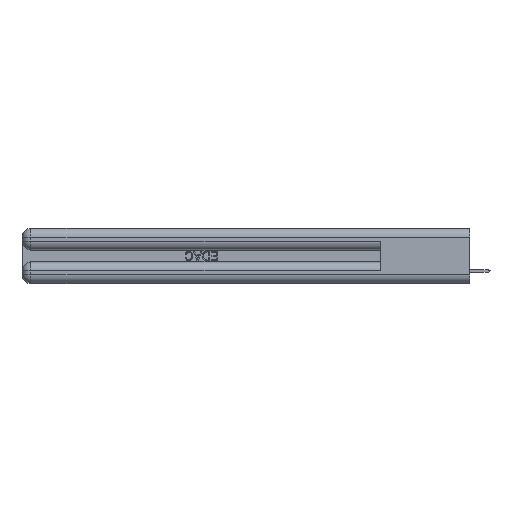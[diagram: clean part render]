
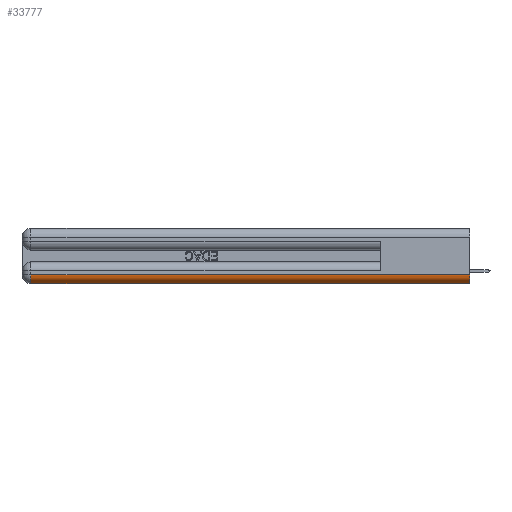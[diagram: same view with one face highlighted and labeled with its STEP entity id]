
A CAD part, left-side view. The second image highlights one B-rep face of the part: STEP entity #33777.
In plain terms, the highlighted cylindrical face has radius 1.524 mm (diameter 3.048 mm), a partial arc.
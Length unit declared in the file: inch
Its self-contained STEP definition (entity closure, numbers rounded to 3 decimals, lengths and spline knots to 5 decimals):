
#1244 = VERTEX_POINT ( 'NONE', #5500 ) ;
#2413 = CARTESIAN_POINT ( 'NONE',  ( 0., 0., 0.06 ) ) ;
#3507 = VERTEX_POINT ( 'NONE', #13268 ) ;
#4383 = EDGE_CURVE ( 'NONE', #1244, #14507, #7246, .T. ) ;
#5500 = CARTESIAN_POINT ( 'NONE',  ( 0., 2.94, 0.06 ) ) ;
#5751 = CIRCLE ( 'NONE', #48124, 0.06 ) ;
#5882 = EDGE_CURVE ( 'NONE', #14507, #11333, #44890, .T. ) ;
#7246 = LINE ( 'NONE', #2413, #22375 ) ;
#7659 = CARTESIAN_POINT ( 'NONE',  ( 0.06, 2.94, 0.06 ) ) ;
#11333 = VERTEX_POINT ( 'NONE', #26010 ) ;
#11801 = CARTESIAN_POINT ( 'NONE',  ( 0.06, 0., 0.06 ) ) ;
#12613 = CARTESIAN_POINT ( 'NONE',  ( 0.06, 3., 0. ) ) ;
#12661 = CARTESIAN_POINT ( 'NONE',  ( 0., 0., 0.06 ) ) ;
#13268 = CARTESIAN_POINT ( 'NONE',  ( 0.06, 2.94, 0. ) ) ;
#14507 = VERTEX_POINT ( 'NONE', #12661 ) ;
#19885 = DIRECTION ( 'NONE',  ( 0., 1., 0. ) ) ;
#19975 = DIRECTION ( 'NONE',  ( 0., -1., 0. ) ) ;
#21925 = EDGE_LOOP ( 'NONE', ( #24164, #37095, #25626, #23509 ) ) ;
#22375 = VECTOR ( 'NONE', #50115, 39.37008 ) ;
#22393 = AXIS2_PLACEMENT_3D ( 'NONE', #49402, #38197, #22598 ) ;
#22598 = DIRECTION ( 'NONE',  ( 0., 0., 1. ) ) ;
#23509 = ORIENTED_EDGE ( 'NONE', *, *, #40601, .F. ) ;
#24164 = ORIENTED_EDGE ( 'NONE', *, *, #5882, .F. ) ;
#25626 = ORIENTED_EDGE ( 'NONE', *, *, #44411, .F. ) ;
#26010 = CARTESIAN_POINT ( 'NONE',  ( 0.06, 0., 0. ) ) ;
#29277 = VECTOR ( 'NONE', #43828, 39.37008 ) ;
#31761 = DIRECTION ( 'NONE',  ( 0., 0., 1. ) ) ;
#33777 = ADVANCED_FACE ( 'NONE', ( #45344 ), #34359, .T. ) ;
#34359 = CYLINDRICAL_SURFACE ( 'NONE', #22393, 0.06 ) ;
#37095 = ORIENTED_EDGE ( 'NONE', *, *, #4383, .F. ) ;
#38197 = DIRECTION ( 'NONE',  ( 0., 1., 0. ) ) ;
#39975 = LINE ( 'NONE', #12613, #29277 ) ;
#40601 = EDGE_CURVE ( 'NONE', #11333, #3507, #39975, .T. ) ;
#42899 = DIRECTION ( 'NONE',  ( 0., 0., 1. ) ) ;
#43828 = DIRECTION ( 'NONE',  ( 0., 1., 0. ) ) ;
#44411 = EDGE_CURVE ( 'NONE', #3507, #1244, #5751, .T. ) ;
#44890 = CIRCLE ( 'NONE', #49798, 0.06 ) ;
#45344 = FACE_OUTER_BOUND ( 'NONE', #21925, .T. ) ;
#48124 = AXIS2_PLACEMENT_3D ( 'NONE', #7659, #19885, #42899 ) ;
#49402 = CARTESIAN_POINT ( 'NONE',  ( 0.06, 0., 0.06 ) ) ;
#49798 = AXIS2_PLACEMENT_3D ( 'NONE', #11801, #19975, #31761 ) ;
#50115 = DIRECTION ( 'NONE',  ( 0., -1., 0. ) ) ;
